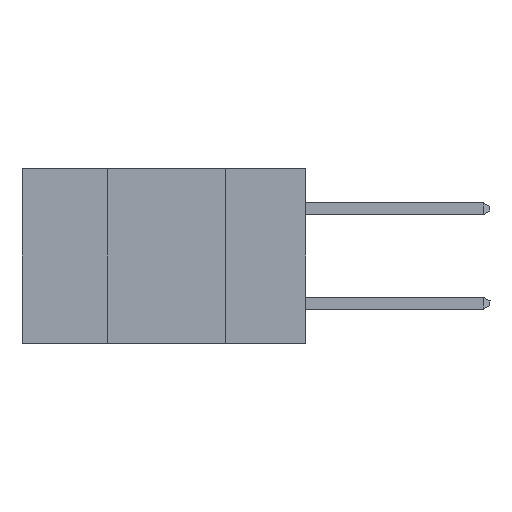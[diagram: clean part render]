
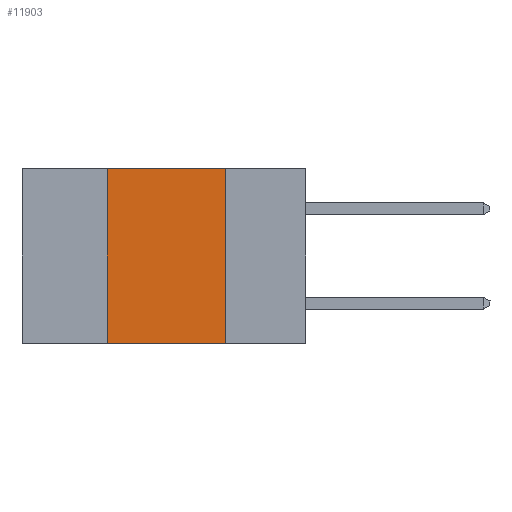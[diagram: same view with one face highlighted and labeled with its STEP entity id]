
A CAD part, left-side view. The second image highlights one B-rep face of the part: STEP entity #11903.
In plain terms, the highlighted planar face has unit normal (-1, 0, 0).
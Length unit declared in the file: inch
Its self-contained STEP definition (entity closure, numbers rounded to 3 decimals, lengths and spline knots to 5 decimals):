
#506 = PLANE ( 'NONE',  #3245 ) ;
#2467 = DIRECTION ( 'NONE',  ( 0., -1., 0. ) ) ;
#2723 = VECTOR ( 'NONE', #7313, 39.37008 ) ;
#2821 = VERTEX_POINT ( 'NONE', #11849 ) ;
#3033 = CARTESIAN_POINT ( 'NONE',  ( 0., 0.42, 0. ) ) ;
#3042 = CARTESIAN_POINT ( 'NONE',  ( 0., 0.17, 0. ) ) ;
#3245 = AXIS2_PLACEMENT_3D ( 'NONE', #12241, #10135, #5862 ) ;
#3295 = EDGE_CURVE ( 'NONE', #5866, #7215, #4077, .T. ) ;
#4077 = LINE ( 'NONE', #13604, #13297 ) ;
#4087 = EDGE_CURVE ( 'NONE', #7215, #2821, #11438, .T. ) ;
#4439 = EDGE_LOOP ( 'NONE', ( #7805, #11230, #13552, #12730 ) ) ;
#4840 = LINE ( 'NONE', #7208, #11362 ) ;
#5696 = CARTESIAN_POINT ( 'NONE',  ( 0., 0.17, 0. ) ) ;
#5862 = DIRECTION ( 'NONE',  ( 0., 0., -1. ) ) ;
#5866 = VERTEX_POINT ( 'NONE', #3033 ) ;
#6127 = DIRECTION ( 'NONE',  ( 0., 0., 1. ) ) ;
#6692 = EDGE_CURVE ( 'NONE', #9019, #5866, #4840, .T. ) ;
#7208 = CARTESIAN_POINT ( 'NONE',  ( 0., 0.42, 0. ) ) ;
#7215 = VERTEX_POINT ( 'NONE', #5696 ) ;
#7313 = DIRECTION ( 'NONE',  ( 0., 0., -1. ) ) ;
#7339 = DIRECTION ( 'NONE',  ( 0., -1., 0. ) ) ;
#7805 = ORIENTED_EDGE ( 'NONE', *, *, #4087, .F. ) ;
#8420 = CARTESIAN_POINT ( 'NONE',  ( 0., 0.42, -0.37 ) ) ;
#9019 = VERTEX_POINT ( 'NONE', #8420 ) ;
#10036 = CARTESIAN_POINT ( 'NONE',  ( 0., 0.6, -0.37 ) ) ;
#10135 = DIRECTION ( 'NONE',  ( 1., 0., 0. ) ) ;
#11230 = ORIENTED_EDGE ( 'NONE', *, *, #3295, .F. ) ;
#11362 = VECTOR ( 'NONE', #6127, 39.37008 ) ;
#11438 = LINE ( 'NONE', #3042, #2723 ) ;
#11649 = FACE_OUTER_BOUND ( 'NONE', #4439, .T. ) ;
#11838 = LINE ( 'NONE', #10036, #13668 ) ;
#11849 = CARTESIAN_POINT ( 'NONE',  ( 0., 0.17, -0.37 ) ) ;
#11903 = ADVANCED_FACE ( 'NONE', ( #11649 ), #506, .F. ) ;
#12241 = CARTESIAN_POINT ( 'NONE',  ( 0., 0.6, 0. ) ) ;
#12730 = ORIENTED_EDGE ( 'NONE', *, *, #13071, .T. ) ;
#13071 = EDGE_CURVE ( 'NONE', #9019, #2821, #11838, .T. ) ;
#13297 = VECTOR ( 'NONE', #7339, 39.37008 ) ;
#13552 = ORIENTED_EDGE ( 'NONE', *, *, #6692, .F. ) ;
#13604 = CARTESIAN_POINT ( 'NONE',  ( 0., 0.6, 0. ) ) ;
#13668 = VECTOR ( 'NONE', #2467, 39.37008 ) ;
